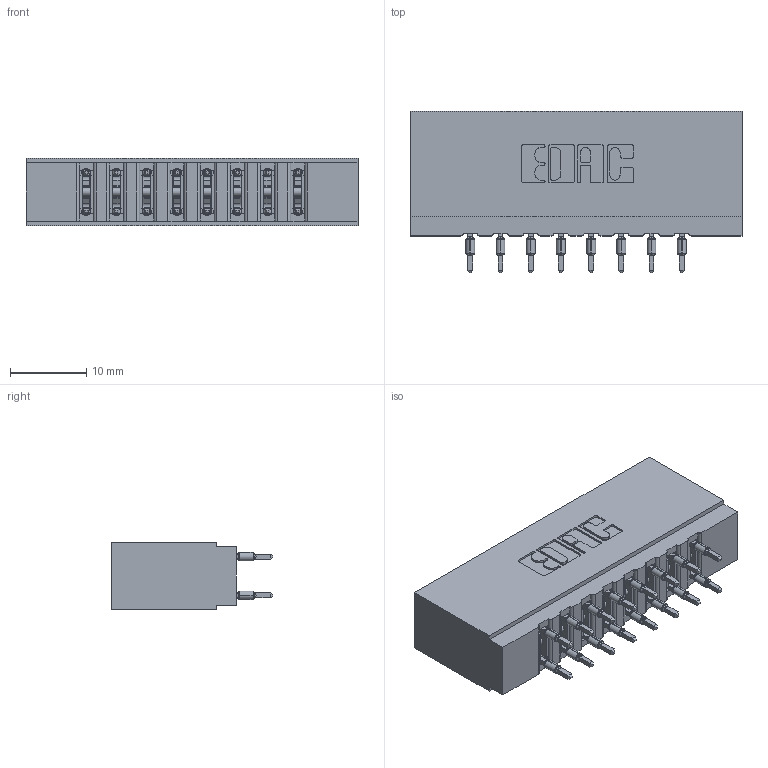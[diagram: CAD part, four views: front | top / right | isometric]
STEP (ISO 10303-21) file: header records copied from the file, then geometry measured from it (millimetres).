
FILE_DESCRIPTION (( 'STEP AP203' ), '1' );
FILE_NAME ('737-016-560-201.STEP', '2020-09-10T20:10:30', ( '' ), ( '' ), 'SwSTEP 2.0', 'SolidWorks 2020', '' );
FILE_SCHEMA (( 'CONFIG_CONTROL_DESIGN' ));
Length unit declared in the file: inch
Products named in the file (3): 737 Part_Insulator Option - 01; 745-292-001_560; 737-016-560-201
Assembly tree (17 placements, depth 2):
  737-016-560-201
    737 Part_Insulator Option - 01
    745-292-001_560  x16
Bounding box: 43.54 x 21.22 x 8.89 mm (x, y, z)
Volume: 4578.4 mm3; surface area: 6180.5 mm2
Topology: 17 solids, 17 shells, 1678 faces, 4591 edges, 2922 vertices
Faces by surface type: plane 878, cylinder 384, bspline 320, torus 96
Entity records: 18670 total; most frequent: CARTESIAN_POINT 3755, ORIENTED_EDGE 3122, DIRECTION 2759, EDGE_CURVE 1561, VECTOR 1323, LINE 1323, VERTEX_POINT 1002, AXIS2_PLACEMENT_3D 718
